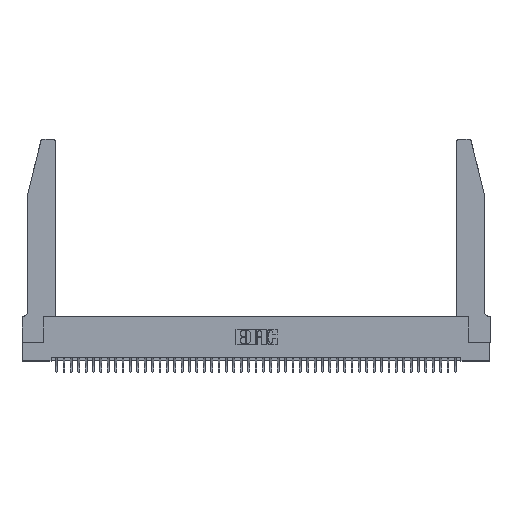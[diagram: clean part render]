
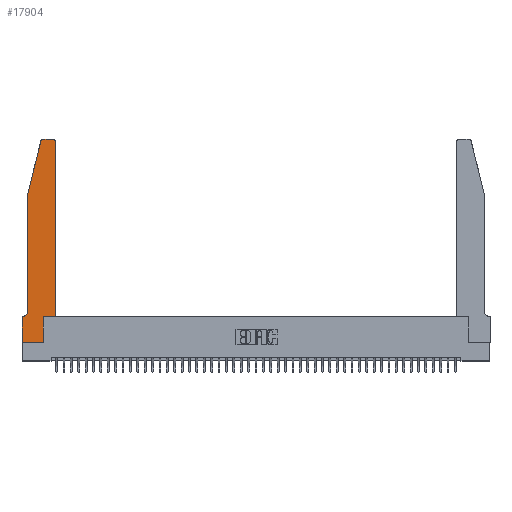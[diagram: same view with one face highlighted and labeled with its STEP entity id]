
A CAD part, top view. The second image highlights one B-rep face of the part: STEP entity #17904.
In plain terms, the highlighted planar face has unit normal (0, 0, 1).
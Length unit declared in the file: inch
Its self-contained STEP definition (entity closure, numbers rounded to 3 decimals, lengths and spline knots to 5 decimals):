
#746 = EDGE_CURVE ( 'NONE', #33931, #8587, #34877, .T. ) ;
#1017 = DIRECTION ( 'NONE',  ( 1., 0., 0. ) ) ;
#1423 = CARTESIAN_POINT ( 'NONE',  ( 0.0755, 0.35, 0.37 ) ) ;
#1778 = VECTOR ( 'NONE', #34099, 39.37008 ) ;
#1836 = PLANE ( 'NONE',  #44794 ) ;
#2434 = VERTEX_POINT ( 'NONE', #22486 ) ;
#2870 = CARTESIAN_POINT ( 'NONE',  ( 0.4205, 2.72, 0.37 ) ) ;
#2945 = AXIS2_PLACEMENT_3D ( 'NONE', #37050, #32954, #1017 ) ;
#3228 = CIRCLE ( 'NONE', #14944, 0.07 ) ;
#3304 = CARTESIAN_POINT ( 'NONE',  ( 0.0055, 0.42, 0.37 ) ) ;
#4247 = ORIENTED_EDGE ( 'NONE', *, *, #21552, .T. ) ;
#4458 = EDGE_CURVE ( 'NONE', #10882, #33931, #15883, .T. ) ;
#4559 = DIRECTION ( 'NONE',  ( 0., -1., 0. ) ) ;
#4783 = DIRECTION ( 'NONE',  ( 1., 0., 0. ) ) ;
#5112 = DIRECTION ( 'NONE',  ( 1., 0., 0. ) ) ;
#5177 = CARTESIAN_POINT ( 'NONE',  ( 0.2865, 0.35, 0.37 ) ) ;
#5227 = LINE ( 'NONE', #7265, #44346 ) ;
#5545 = LINE ( 'NONE', #19418, #37480 ) ;
#6351 = VECTOR ( 'NONE', #5112, 39.37008 ) ;
#6370 = ORIENTED_EDGE ( 'NONE', *, *, #28394, .T. ) ;
#6514 = CARTESIAN_POINT ( 'NONE',  ( 0.4505, 0.35, 0.37 ) ) ;
#7265 = CARTESIAN_POINT ( 'NONE',  ( 0., 0., 0.37 ) ) ;
#7518 = ORIENTED_EDGE ( 'NONE', *, *, #24913, .T. ) ;
#7646 = DIRECTION ( 'NONE',  ( 1., 0., 0. ) ) ;
#7795 = DIRECTION ( 'NONE',  ( 0., 0., 1. ) ) ;
#8411 = FACE_OUTER_BOUND ( 'NONE', #34103, .T. ) ;
#8587 = VERTEX_POINT ( 'NONE', #32637 ) ;
#8709 = CARTESIAN_POINT ( 'NONE',  ( 0.0755, 2., 0.37 ) ) ;
#8841 = VERTEX_POINT ( 'NONE', #28445 ) ;
#9606 = ORIENTED_EDGE ( 'NONE', *, *, #746, .T. ) ;
#9805 = CARTESIAN_POINT ( 'NONE',  ( 0.284, 2.75, 0.37 ) ) ;
#10542 = DIRECTION ( 'NONE',  ( 0., 0., -1. ) ) ;
#10882 = VERTEX_POINT ( 'NONE', #12492 ) ;
#10907 = ORIENTED_EDGE ( 'NONE', *, *, #11958, .T. ) ;
#10952 = VERTEX_POINT ( 'NONE', #19606 ) ;
#11128 = ORIENTED_EDGE ( 'NONE', *, *, #29791, .T. ) ;
#11283 = DIRECTION ( 'NONE',  ( -1., 0., 0. ) ) ;
#11402 = CARTESIAN_POINT ( 'NONE',  ( 0., 0., 0.37 ) ) ;
#11685 = CARTESIAN_POINT ( 'NONE',  ( 0., 0.35, 0.37 ) ) ;
#11752 = CARTESIAN_POINT ( 'NONE',  ( 0.0755, 2., 0.37 ) ) ;
#11958 = EDGE_CURVE ( 'NONE', #28160, #8841, #35782, .T. ) ;
#12492 = CARTESIAN_POINT ( 'NONE',  ( 0., 0., 0.37 ) ) ;
#12564 = DIRECTION ( 'NONE',  ( -1., 0., 0. ) ) ;
#12700 = EDGE_CURVE ( 'NONE', #10952, #37788, #3228, .T. ) ;
#12895 = DIRECTION ( 'NONE',  ( 0., 1., 0. ) ) ;
#14944 = AXIS2_PLACEMENT_3D ( 'NONE', #3304, #10542, #11283 ) ;
#15022 = CARTESIAN_POINT ( 'NONE',  ( 0.2865, 0., 0.37 ) ) ;
#15847 = VECTOR ( 'NONE', #41361, 39.37008 ) ;
#15883 = LINE ( 'NONE', #11402, #6351 ) ;
#16561 = LINE ( 'NONE', #6514, #34447 ) ;
#17134 = ORIENTED_EDGE ( 'NONE', *, *, #17310, .T. ) ;
#17287 = DIRECTION ( 'NONE',  ( 0., 0., 1. ) ) ;
#17310 = EDGE_CURVE ( 'NONE', #28941, #23780, #21795, .T. ) ;
#17904 = ADVANCED_FACE ( 'NONE', ( #8411 ), #1836, .T. ) ;
#18875 = DIRECTION ( 'NONE',  ( 0., -1., 0. ) ) ;
#19418 = CARTESIAN_POINT ( 'NONE',  ( 0.2605, 2.75, 0.37 ) ) ;
#19606 = CARTESIAN_POINT ( 'NONE',  ( 0.0755, 0.42, 0.37 ) ) ;
#20119 = ORIENTED_EDGE ( 'NONE', *, *, #4458, .T. ) ;
#21552 = EDGE_CURVE ( 'NONE', #8841, #23646, #41618, .T. ) ;
#21737 = LINE ( 'NONE', #34334, #30750 ) ;
#21795 = CIRCLE ( 'NONE', #24066, 0.03 ) ;
#22486 = CARTESIAN_POINT ( 'NONE',  ( 0.4505, 0.35, 0.37 ) ) ;
#22780 = LINE ( 'NONE', #1423, #44093 ) ;
#23646 = VERTEX_POINT ( 'NONE', #40576 ) ;
#23780 = VERTEX_POINT ( 'NONE', #30438 ) ;
#24066 = AXIS2_PLACEMENT_3D ( 'NONE', #2870, #17287, #7646 ) ;
#24407 = ORIENTED_EDGE ( 'NONE', *, *, #40484, .T. ) ;
#24907 = CARTESIAN_POINT ( 'NONE',  ( 0.4505, 2.72, 0.37 ) ) ;
#24913 = EDGE_CURVE ( 'NONE', #2434, #28941, #21737, .T. ) ;
#26178 = DIRECTION ( 'NONE',  ( -1., 0., 0. ) ) ;
#27523 = ORIENTED_EDGE ( 'NONE', *, *, #28575, .T. ) ;
#28014 = CARTESIAN_POINT ( 'NONE',  ( 0.0055, 0.35, 0.37 ) ) ;
#28160 = VERTEX_POINT ( 'NONE', #9805 ) ;
#28200 = EDGE_CURVE ( 'NONE', #8587, #2434, #16561, .T. ) ;
#28394 = EDGE_CURVE ( 'NONE', #36574, #10882, #5227, .T. ) ;
#28445 = CARTESIAN_POINT ( 'NONE',  ( 0.25487, 2.72718, 0.37 ) ) ;
#28575 = EDGE_CURVE ( 'NONE', #23780, #28160, #5545, .T. ) ;
#28941 = VERTEX_POINT ( 'NONE', #24907 ) ;
#29791 = EDGE_CURVE ( 'NONE', #23646, #10952, #34571, .T. ) ;
#30438 = CARTESIAN_POINT ( 'NONE',  ( 0.4205, 2.75, 0.37 ) ) ;
#30750 = VECTOR ( 'NONE', #12895, 39.37008 ) ;
#32080 = ORIENTED_EDGE ( 'NONE', *, *, #12700, .T. ) ;
#32637 = CARTESIAN_POINT ( 'NONE',  ( 0.2865, 0.35, 0.37 ) ) ;
#32954 = DIRECTION ( 'NONE',  ( 0., 0., 1. ) ) ;
#33931 = VERTEX_POINT ( 'NONE', #15022 ) ;
#34099 = DIRECTION ( 'NONE',  ( -0.239, -0.971, 0. ) ) ;
#34103 = EDGE_LOOP ( 'NONE', ( #27523, #10907, #4247, #11128, #32080, #24407, #6370, #20119, #9606, #45193, #7518, #17134 ) ) ;
#34334 = CARTESIAN_POINT ( 'NONE',  ( 0.4505, 0.35, 0.37 ) ) ;
#34447 = VECTOR ( 'NONE', #42059, 39.37008 ) ;
#34571 = LINE ( 'NONE', #8709, #41321 ) ;
#34877 = LINE ( 'NONE', #5177, #15847 ) ;
#35782 = CIRCLE ( 'NONE', #2945, 0.03 ) ;
#36574 = VERTEX_POINT ( 'NONE', #11685 ) ;
#37050 = CARTESIAN_POINT ( 'NONE',  ( 0.284, 2.72, 0.37 ) ) ;
#37480 = VECTOR ( 'NONE', #12564, 39.37008 ) ;
#37788 = VERTEX_POINT ( 'NONE', #28014 ) ;
#40484 = EDGE_CURVE ( 'NONE', #37788, #36574, #22780, .T. ) ;
#40576 = CARTESIAN_POINT ( 'NONE',  ( 0.0755, 2., 0.37 ) ) ;
#41321 = VECTOR ( 'NONE', #18875, 39.37008 ) ;
#41361 = DIRECTION ( 'NONE',  ( 0., 1., 0. ) ) ;
#41618 = LINE ( 'NONE', #11752, #1778 ) ;
#42059 = DIRECTION ( 'NONE',  ( 1., 0., 0. ) ) ;
#44093 = VECTOR ( 'NONE', #26178, 39.37008 ) ;
#44346 = VECTOR ( 'NONE', #4559, 39.37008 ) ;
#44794 = AXIS2_PLACEMENT_3D ( 'NONE', #46176, #7795, #4783 ) ;
#45193 = ORIENTED_EDGE ( 'NONE', *, *, #28200, .T. ) ;
#46176 = CARTESIAN_POINT ( 'NONE',  ( 0., 0.35, 0.37 ) ) ;
